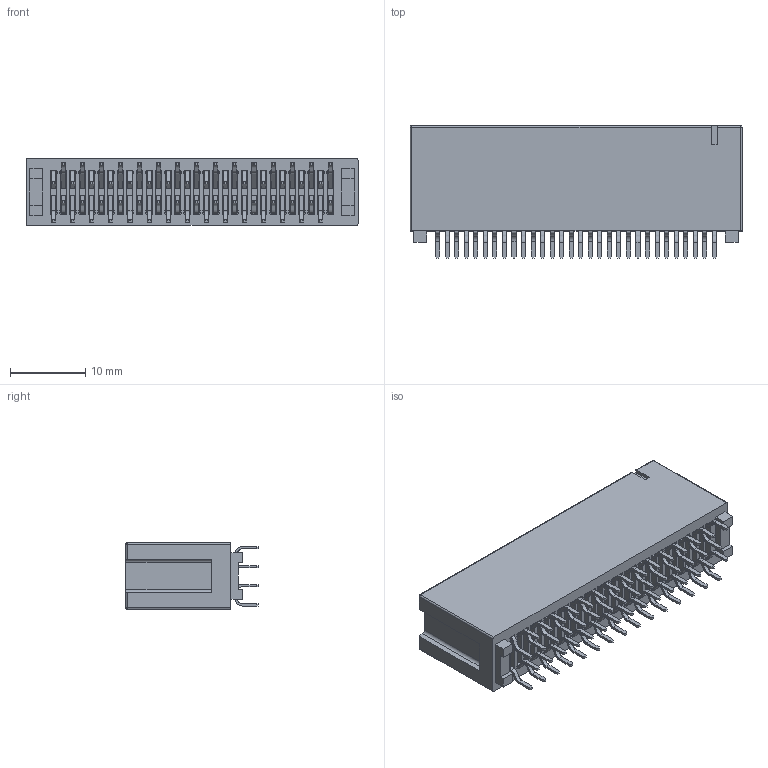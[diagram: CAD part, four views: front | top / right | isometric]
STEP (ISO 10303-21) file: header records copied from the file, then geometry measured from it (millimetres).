
FILE_DESCRIPTION (( 'STEP AP203' ), '1' );
FILE_NAME ('302-060-621-201.STEP', '2024-03-28T20:45:01', ( '' ), ( '' ), 'SwSTEP 2.0', 'SolidWorks 2023', '' );
FILE_SCHEMA (( 'CONFIG_CONTROL_DESIGN' ));
Length unit declared in the file: millimetre
Products named in the file (4): Contact_302-290-X21 (1); 302-060-621-201; Contact_302-290-X21 (2); HSG_Vertical HSG
Assembly tree (61 placements, depth 2):
  302-060-621-201
    HSG_Vertical HSG
    Contact_302-290-X21 (2)  x30
    Contact_302-290-X21 (1)  x30
Bounding box: 44.2 x 17.63 x 8.88 mm (x, y, z)
Volume: 3464.4 mm3; surface area: 9307.1 mm2
Topology: 61 solids, 61 shells, 2796 faces, 8208 edges, 5384 vertices
Faces by surface type: plane 2059, cylinder 613, bspline 120, sphere 4
Entity records: 25436 total; most frequent: CARTESIAN_POINT 4372, ORIENTED_EDGE 4344, DIRECTION 3534, EDGE_CURVE 2172, VECTOR 2098, LINE 2098, VERTEX_POINT 1440, AXIS2_PLACEMENT_3D 718
